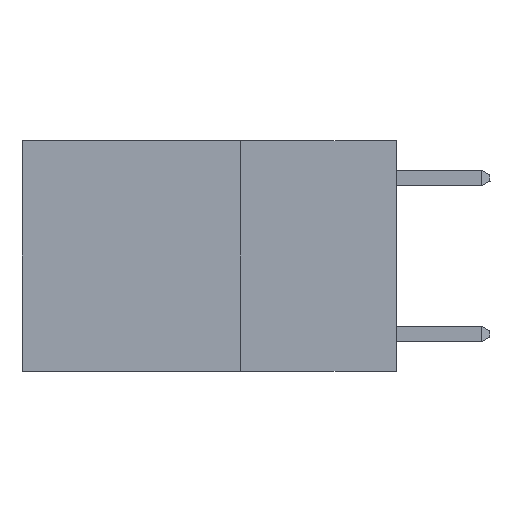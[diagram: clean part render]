
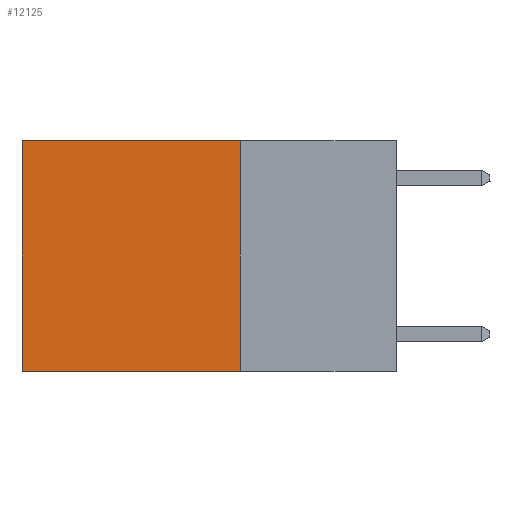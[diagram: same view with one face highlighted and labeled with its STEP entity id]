
A CAD part, left-side view. The second image highlights one B-rep face of the part: STEP entity #12125.
In plain terms, the highlighted planar face has unit normal (-1, 0, 0).
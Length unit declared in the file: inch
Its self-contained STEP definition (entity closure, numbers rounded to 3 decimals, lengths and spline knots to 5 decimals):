
#113 = LINE ( 'NONE', #10845, #13719 ) ;
#655 = ORIENTED_EDGE ( 'NONE', *, *, #13335, .F. ) ;
#803 = CARTESIAN_POINT ( 'NONE',  ( 0.2625, 0.25, -0.37 ) ) ;
#2727 = LINE ( 'NONE', #16273, #16347 ) ;
#3250 = PLANE ( 'NONE',  #12511 ) ;
#3304 = LINE ( 'NONE', #6114, #4536 ) ;
#3366 = DIRECTION ( 'NONE',  ( 1., 0., 0. ) ) ;
#3549 = DIRECTION ( 'NONE',  ( 0., 1., 0. ) ) ;
#3864 = ORIENTED_EDGE ( 'NONE', *, *, #12064, .T. ) ;
#4536 = VECTOR ( 'NONE', #3549, 39.37008 ) ;
#5539 = CARTESIAN_POINT ( 'NONE',  ( 0.2625, 0.6, 0. ) ) ;
#5940 = CARTESIAN_POINT ( 'NONE',  ( 0.2625, 0.6, -0.37 ) ) ;
#6002 = DIRECTION ( 'NONE',  ( 0., 0., -1. ) ) ;
#6026 = DIRECTION ( 'NONE',  ( 0., 0., -1. ) ) ;
#6034 = VERTEX_POINT ( 'NONE', #803 ) ;
#6114 = CARTESIAN_POINT ( 'NONE',  ( 0.2625, 0.25, -0.37 ) ) ;
#6898 = FACE_OUTER_BOUND ( 'NONE', #9398, .T. ) ;
#8409 = CARTESIAN_POINT ( 'NONE',  ( 0.2625, 0.25, 0. ) ) ;
#8446 = CARTESIAN_POINT ( 'NONE',  ( 0.2625, 0.25, 0. ) ) ;
#8472 = EDGE_CURVE ( 'NONE', #10174, #15710, #12851, .T. ) ;
#8800 = ORIENTED_EDGE ( 'NONE', *, *, #9908, .F. ) ;
#9227 = VERTEX_POINT ( 'NONE', #8409 ) ;
#9307 = ORIENTED_EDGE ( 'NONE', *, *, #8472, .T. ) ;
#9398 = EDGE_LOOP ( 'NONE', ( #9307, #8800, #655, #3864 ) ) ;
#9908 = EDGE_CURVE ( 'NONE', #6034, #15710, #3304, .T. ) ;
#10174 = VERTEX_POINT ( 'NONE', #5539 ) ;
#10845 = CARTESIAN_POINT ( 'NONE',  ( 0.2625, 0.25, 0. ) ) ;
#11427 = DIRECTION ( 'NONE',  ( 0., 0., -1. ) ) ;
#12064 = EDGE_CURVE ( 'NONE', #9227, #10174, #113, .T. ) ;
#12125 = ADVANCED_FACE ( 'NONE', ( #6898 ), #3250, .F. ) ;
#12511 = AXIS2_PLACEMENT_3D ( 'NONE', #8446, #3366, #6026 ) ;
#12851 = LINE ( 'NONE', #14164, #16568 ) ;
#13335 = EDGE_CURVE ( 'NONE', #9227, #6034, #2727, .T. ) ;
#13719 = VECTOR ( 'NONE', #13801, 39.37008 ) ;
#13801 = DIRECTION ( 'NONE',  ( 0., 1., 0. ) ) ;
#14164 = CARTESIAN_POINT ( 'NONE',  ( 0.2625, 0.6, 0. ) ) ;
#15710 = VERTEX_POINT ( 'NONE', #5940 ) ;
#16273 = CARTESIAN_POINT ( 'NONE',  ( 0.2625, 0.25, 0. ) ) ;
#16347 = VECTOR ( 'NONE', #6002, 39.37008 ) ;
#16568 = VECTOR ( 'NONE', #11427, 39.37008 ) ;
